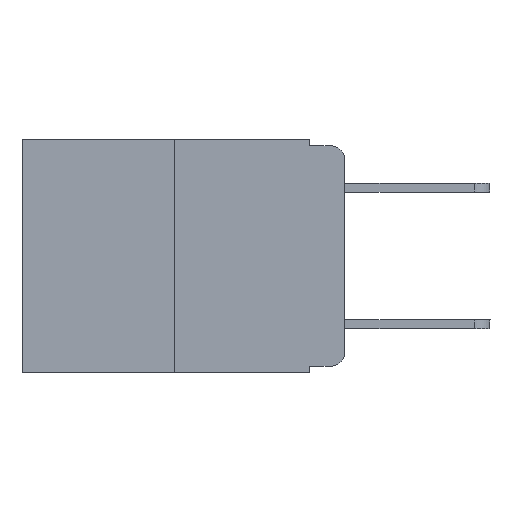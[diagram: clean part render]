
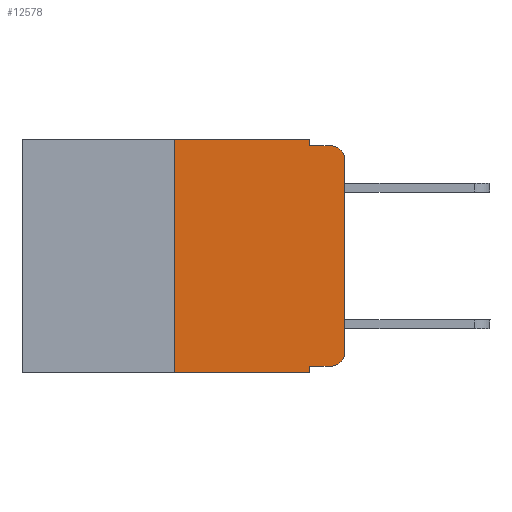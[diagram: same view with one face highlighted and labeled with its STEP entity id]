
A CAD part, left-side view. The second image highlights one B-rep face of the part: STEP entity #12578.
In plain terms, the highlighted planar face has unit normal (-1, 0, 0).
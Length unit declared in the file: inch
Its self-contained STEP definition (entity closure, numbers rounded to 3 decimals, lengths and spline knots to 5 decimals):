
#86 = VERTEX_POINT ( 'NONE', #7720 ) ;
#130 = CARTESIAN_POINT ( 'NONE',  ( 0., 0.473, 0. ) ) ;
#730 = EDGE_CURVE ( 'NONE', #6917, #10302, #12385, .T. ) ;
#900 = CARTESIAN_POINT ( 'NONE',  ( 0., 0.051, 0. ) ) ;
#1495 = VECTOR ( 'NONE', #2269, 39.37008 ) ;
#1508 = VECTOR ( 'NONE', #13950, 39.37008 ) ;
#1887 = CARTESIAN_POINT ( 'NONE',  ( 0., 0.02, -0.313 ) ) ;
#1939 = AXIS2_PLACEMENT_3D ( 'NONE', #1887, #16543, #19940 ) ;
#2132 = ORIENTED_EDGE ( 'NONE', *, *, #6074, .F. ) ;
#2269 = DIRECTION ( 'NONE',  ( 0., 0., -1. ) ) ;
#2340 = CARTESIAN_POINT ( 'NONE',  ( 0., 0.051, 0. ) ) ;
#2391 = CARTESIAN_POINT ( 'NONE',  ( 0., 0.473, 0. ) ) ;
#2568 = CARTESIAN_POINT ( 'NONE',  ( 0., 0., -0.313 ) ) ;
#3441 = ORIENTED_EDGE ( 'NONE', *, *, #730, .T. ) ;
#3917 = ORIENTED_EDGE ( 'NONE', *, *, #9900, .F. ) ;
#4153 = EDGE_CURVE ( 'NONE', #20440, #15232, #19007, .T. ) ;
#4252 = VERTEX_POINT ( 'NONE', #2568 ) ;
#5231 = DIRECTION ( 'NONE',  ( 0., -1., 0. ) ) ;
#5410 = ORIENTED_EDGE ( 'NONE', *, *, #16615, .T. ) ;
#5975 = CARTESIAN_POINT ( 'NONE',  ( 0., 0.02, -0.01 ) ) ;
#6074 = EDGE_CURVE ( 'NONE', #86, #18368, #9365, .T. ) ;
#6254 = DIRECTION ( 'NONE',  ( 0., -1., 0. ) ) ;
#6757 = CARTESIAN_POINT ( 'NONE',  ( 0., 0., -0.03 ) ) ;
#6917 = VERTEX_POINT ( 'NONE', #7385 ) ;
#7367 = DIRECTION ( 'NONE',  ( 1., 0., 0. ) ) ;
#7385 = CARTESIAN_POINT ( 'NONE',  ( 0., 0.051, -0.333 ) ) ;
#7582 = DIRECTION ( 'NONE',  ( 0., 0., -1. ) ) ;
#7720 = CARTESIAN_POINT ( 'NONE',  ( 0., 0.25, -0.343 ) ) ;
#7875 = EDGE_CURVE ( 'NONE', #10302, #4252, #18039, .T. ) ;
#8021 = AXIS2_PLACEMENT_3D ( 'NONE', #14807, #16472, #9951 ) ;
#8326 = ORIENTED_EDGE ( 'NONE', *, *, #7875, .T. ) ;
#8367 = ORIENTED_EDGE ( 'NONE', *, *, #14397, .F. ) ;
#8520 = VECTOR ( 'NONE', #6254, 39.37008 ) ;
#8599 = CARTESIAN_POINT ( 'NONE',  ( 0., 0.051, -0.343 ) ) ;
#9365 = LINE ( 'NONE', #16878, #14229 ) ;
#9900 = EDGE_CURVE ( 'NONE', #6917, #20362, #20528, .T. ) ;
#9951 = DIRECTION ( 'NONE',  ( 0., 0., -1. ) ) ;
#9974 = DIRECTION ( 'NONE',  ( 0., 0., 1. ) ) ;
#10302 = VERTEX_POINT ( 'NONE', #16055 ) ;
#10397 = LINE ( 'NONE', #19821, #11676 ) ;
#10608 = PLANE ( 'NONE',  #16613 ) ;
#11139 = CIRCLE ( 'NONE', #8021, 0.02 ) ;
#11522 = VERTEX_POINT ( 'NONE', #5975 ) ;
#11676 = VECTOR ( 'NONE', #9974, 39.37008 ) ;
#12012 = LINE ( 'NONE', #19545, #16081 ) ;
#12385 = LINE ( 'NONE', #17984, #8520 ) ;
#12578 = ADVANCED_FACE ( 'NONE', ( #17188 ), #10608, .F. ) ;
#13274 = VECTOR ( 'NONE', #13679, 39.37008 ) ;
#13333 = CARTESIAN_POINT ( 'NONE',  ( 0., 0.051, -0.01 ) ) ;
#13373 = CARTESIAN_POINT ( 'NONE',  ( 0., 0.051, -0.01 ) ) ;
#13679 = DIRECTION ( 'NONE',  ( 0., -1., 0. ) ) ;
#13950 = DIRECTION ( 'NONE',  ( 0., 0., -1. ) ) ;
#13988 = ORIENTED_EDGE ( 'NONE', *, *, #14124, .T. ) ;
#14124 = EDGE_CURVE ( 'NONE', #86, #20362, #12012, .T. ) ;
#14203 = EDGE_LOOP ( 'NONE', ( #15306, #5410, #8367, #18189, #14480, #2132, #13988, #3917, #3441, #8326 ) ) ;
#14229 = VECTOR ( 'NONE', #16810, 39.37008 ) ;
#14274 = VECTOR ( 'NONE', #5231, 39.37008 ) ;
#14303 = EDGE_CURVE ( 'NONE', #18368, #20440, #16854, .T. ) ;
#14397 = EDGE_CURVE ( 'NONE', #15232, #11522, #17107, .T. ) ;
#14480 = ORIENTED_EDGE ( 'NONE', *, *, #14303, .F. ) ;
#14807 = CARTESIAN_POINT ( 'NONE',  ( 0., 0.02, -0.03 ) ) ;
#15232 = VERTEX_POINT ( 'NONE', #13373 ) ;
#15306 = ORIENTED_EDGE ( 'NONE', *, *, #15797, .T. ) ;
#15797 = EDGE_CURVE ( 'NONE', #4252, #17977, #10397, .T. ) ;
#16041 = DIRECTION ( 'NONE',  ( 0., -1., 0. ) ) ;
#16055 = CARTESIAN_POINT ( 'NONE',  ( 0., 0.02, -0.333 ) ) ;
#16081 = VECTOR ( 'NONE', #16041, 39.37008 ) ;
#16115 = CARTESIAN_POINT ( 'NONE',  ( 0., 0.25, 0. ) ) ;
#16472 = DIRECTION ( 'NONE',  ( -1., 0., 0. ) ) ;
#16543 = DIRECTION ( 'NONE',  ( -1., 0., 0. ) ) ;
#16613 = AXIS2_PLACEMENT_3D ( 'NONE', #2391, #7367, #7582 ) ;
#16615 = EDGE_CURVE ( 'NONE', #17977, #11522, #11139, .T. ) ;
#16810 = DIRECTION ( 'NONE',  ( 0., 0., 1. ) ) ;
#16854 = LINE ( 'NONE', #130, #14274 ) ;
#16878 = CARTESIAN_POINT ( 'NONE',  ( 0., 0.25, 0. ) ) ;
#16912 = CARTESIAN_POINT ( 'NONE',  ( 0., 0.051, 0. ) ) ;
#17107 = LINE ( 'NONE', #13333, #13274 ) ;
#17188 = FACE_OUTER_BOUND ( 'NONE', #14203, .T. ) ;
#17977 = VERTEX_POINT ( 'NONE', #6757 ) ;
#17984 = CARTESIAN_POINT ( 'NONE',  ( 0., 0.051, -0.333 ) ) ;
#18039 = CIRCLE ( 'NONE', #1939, 0.02 ) ;
#18189 = ORIENTED_EDGE ( 'NONE', *, *, #4153, .F. ) ;
#18368 = VERTEX_POINT ( 'NONE', #16115 ) ;
#19007 = LINE ( 'NONE', #2340, #1495 ) ;
#19545 = CARTESIAN_POINT ( 'NONE',  ( 0., 0.473, -0.343 ) ) ;
#19821 = CARTESIAN_POINT ( 'NONE',  ( 0., 0., 0. ) ) ;
#19940 = DIRECTION ( 'NONE',  ( 0., 0., -1. ) ) ;
#20362 = VERTEX_POINT ( 'NONE', #8599 ) ;
#20440 = VERTEX_POINT ( 'NONE', #16912 ) ;
#20528 = LINE ( 'NONE', #900, #1508 ) ;
